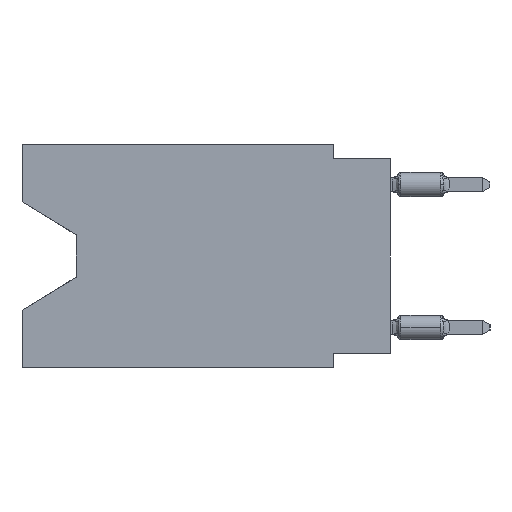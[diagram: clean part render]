
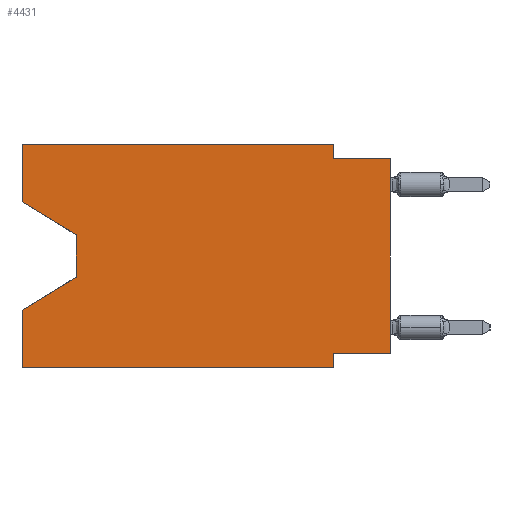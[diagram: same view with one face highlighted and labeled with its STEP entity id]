
A CAD part, left-side view. The second image highlights one B-rep face of the part: STEP entity #4431.
In plain terms, the highlighted planar face has unit normal (-1, 0, 0).
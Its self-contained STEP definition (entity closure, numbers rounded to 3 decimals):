
#127 = ORIENTED_EDGE ( 'NONE', *, *, #1039, .T. ) ;
#1039 = EDGE_CURVE ( 'NONE', #34887, #13111, #49530, .T. ) ;
#1894 = VERTEX_POINT ( 'NONE', #21751 ) ;
#2171 = EDGE_LOOP ( 'NONE', ( #127, #11190, #15120, #26496, #33015, #48427, #23847, #25367, #46181, #34210, #42663, #42930 ) ) ;
#2416 = DIRECTION ( 'NONE',  ( 1., 0., 0. ) ) ;
#3726 = DIRECTION ( 'NONE',  ( 0., -1., 0. ) ) ;
#3860 = VERTEX_POINT ( 'NONE', #38216 ) ;
#4060 = CARTESIAN_POINT ( 'NONE',  ( 0., 13.97, -4.013 ) ) ;
#4105 = CARTESIAN_POINT ( 'NONE',  ( 0., 2.54, -9.906 ) ) ;
#4187 = VECTOR ( 'NONE', #3726, 1000. ) ;
#4391 = VECTOR ( 'NONE', #30835, 1000. ) ;
#4431 = ADVANCED_FACE ( 'NONE', ( #23370 ), #11126, .F. ) ;
#4784 = CARTESIAN_POINT ( 'NONE',  ( 0., 13.97, -4.013 ) ) ;
#5749 = VECTOR ( 'NONE', #38056, 1000. ) ;
#6644 = DIRECTION ( 'NONE',  ( 0., -1., 0. ) ) ;
#7010 = LINE ( 'NONE', #11376, #11803 ) ;
#7080 = EDGE_CURVE ( 'NONE', #3860, #18560, #20617, .T. ) ;
#8147 = DIRECTION ( 'NONE',  ( 0., -0.855, -0.519 ) ) ;
#8660 = DIRECTION ( 'NONE',  ( 0., 0., -1. ) ) ;
#9831 = CARTESIAN_POINT ( 'NONE',  ( 0., 0., -0.635 ) ) ;
#10659 = EDGE_CURVE ( 'NONE', #34887, #3860, #22140, .T. ) ;
#11126 = PLANE ( 'NONE',  #47541 ) ;
#11190 = ORIENTED_EDGE ( 'NONE', *, *, #38778, .T. ) ;
#11282 = CARTESIAN_POINT ( 'NONE',  ( 0., 16.383, -9.906 ) ) ;
#11376 = CARTESIAN_POINT ( 'NONE',  ( 0., 16.383, 0. ) ) ;
#11718 = LINE ( 'NONE', #4060, #34332 ) ;
#11803 = VECTOR ( 'NONE', #48397, 1000. ) ;
#11830 = VECTOR ( 'NONE', #6644, 1000. ) ;
#12264 = VERTEX_POINT ( 'NONE', #4105 ) ;
#12489 = LINE ( 'NONE', #20931, #5749 ) ;
#13111 = VERTEX_POINT ( 'NONE', #4784 ) ;
#13801 = VERTEX_POINT ( 'NONE', #52596 ) ;
#14171 = EDGE_CURVE ( 'NONE', #26111, #46041, #38941, .T. ) ;
#15120 = ORIENTED_EDGE ( 'NONE', *, *, #14171, .T. ) ;
#15475 = CARTESIAN_POINT ( 'NONE',  ( 0., 16.383, 0. ) ) ;
#15873 = LINE ( 'NONE', #32461, #23120 ) ;
#16841 = CARTESIAN_POINT ( 'NONE',  ( 0., 2.54, -9.906 ) ) ;
#17109 = LINE ( 'NONE', #16841, #31672 ) ;
#17131 = EDGE_CURVE ( 'NONE', #46244, #46041, #7010, .T. ) ;
#17999 = DIRECTION ( 'NONE',  ( 0., 0.855, -0.519 ) ) ;
#18350 = EDGE_CURVE ( 'NONE', #13801, #36862, #33402, .T. ) ;
#18560 = VERTEX_POINT ( 'NONE', #50554 ) ;
#19128 = EDGE_CURVE ( 'NONE', #46244, #12264, #44469, .T. ) ;
#20617 = LINE ( 'NONE', #49985, #4187 ) ;
#20931 = CARTESIAN_POINT ( 'NONE',  ( 0., 2.54, 0. ) ) ;
#20972 = VERTEX_POINT ( 'NONE', #25330 ) ;
#21751 = CARTESIAN_POINT ( 'NONE',  ( 0., 2.54, -0.635 ) ) ;
#22140 = LINE ( 'NONE', #43083, #4391 ) ;
#23120 = VECTOR ( 'NONE', #29983, 1000. ) ;
#23370 = FACE_OUTER_BOUND ( 'NONE', #2171, .T. ) ;
#23739 = VECTOR ( 'NONE', #8147, 1000. ) ;
#23847 = ORIENTED_EDGE ( 'NONE', *, *, #39685, .F. ) ;
#23990 = CARTESIAN_POINT ( 'NONE',  ( 0., 16.383, -9.906 ) ) ;
#25330 = CARTESIAN_POINT ( 'NONE',  ( 0., 2.54, -9.271 ) ) ;
#25367 = ORIENTED_EDGE ( 'NONE', *, *, #18350, .T. ) ;
#25546 = CARTESIAN_POINT ( 'NONE',  ( 0., 0., -0.635 ) ) ;
#26111 = VERTEX_POINT ( 'NONE', #52553 ) ;
#26496 = ORIENTED_EDGE ( 'NONE', *, *, #17131, .F. ) ;
#26695 = LINE ( 'NONE', #9831, #41961 ) ;
#26961 = DIRECTION ( 'NONE',  ( 0., -1., 0. ) ) ;
#29853 = EDGE_CURVE ( 'NONE', #1894, #36862, #26695, .T. ) ;
#29983 = DIRECTION ( 'NONE',  ( 0., 1., 0. ) ) ;
#30223 = CARTESIAN_POINT ( 'NONE',  ( 0., 13.97, -5.893 ) ) ;
#30835 = DIRECTION ( 'NONE',  ( 0., 0., 1. ) ) ;
#31672 = VECTOR ( 'NONE', #8660, 1000. ) ;
#32461 = CARTESIAN_POINT ( 'NONE',  ( 0., 0., -9.271 ) ) ;
#32605 = CARTESIAN_POINT ( 'NONE',  ( 0., 0., 0. ) ) ;
#33015 = ORIENTED_EDGE ( 'NONE', *, *, #19128, .T. ) ;
#33178 = CARTESIAN_POINT ( 'NONE',  ( 0., 16.383, -2.546 ) ) ;
#33275 = CARTESIAN_POINT ( 'NONE',  ( 0., 16.383, -7.36 ) ) ;
#33402 = LINE ( 'NONE', #32605, #50920 ) ;
#33812 = EDGE_CURVE ( 'NONE', #20972, #12264, #17109, .T. ) ;
#34210 = ORIENTED_EDGE ( 'NONE', *, *, #35596, .F. ) ;
#34332 = VECTOR ( 'NONE', #49003, 1000. ) ;
#34887 = VERTEX_POINT ( 'NONE', #47721 ) ;
#35596 = EDGE_CURVE ( 'NONE', #18560, #1894, #12489, .T. ) ;
#36862 = VERTEX_POINT ( 'NONE', #25546 ) ;
#38056 = DIRECTION ( 'NONE',  ( 0., 0., -1. ) ) ;
#38216 = CARTESIAN_POINT ( 'NONE',  ( 0., 16.383, 0. ) ) ;
#38778 = EDGE_CURVE ( 'NONE', #13111, #26111, #11718, .T. ) ;
#38941 = LINE ( 'NONE', #30223, #42895 ) ;
#39685 = EDGE_CURVE ( 'NONE', #13801, #20972, #15873, .T. ) ;
#40485 = DIRECTION ( 'NONE',  ( 0., 0., -1. ) ) ;
#41576 = DIRECTION ( 'NONE',  ( 0., 0., 1. ) ) ;
#41961 = VECTOR ( 'NONE', #26961, 1000. ) ;
#42663 = ORIENTED_EDGE ( 'NONE', *, *, #7080, .F. ) ;
#42895 = VECTOR ( 'NONE', #17999, 1000. ) ;
#42930 = ORIENTED_EDGE ( 'NONE', *, *, #10659, .F. ) ;
#43083 = CARTESIAN_POINT ( 'NONE',  ( 0., 16.383, 0. ) ) ;
#44469 = LINE ( 'NONE', #11282, #11830 ) ;
#46041 = VERTEX_POINT ( 'NONE', #33275 ) ;
#46181 = ORIENTED_EDGE ( 'NONE', *, *, #29853, .F. ) ;
#46244 = VERTEX_POINT ( 'NONE', #23990 ) ;
#47541 = AXIS2_PLACEMENT_3D ( 'NONE', #15475, #2416, #40485 ) ;
#47721 = CARTESIAN_POINT ( 'NONE',  ( 0., 16.383, -2.546 ) ) ;
#48397 = DIRECTION ( 'NONE',  ( 0., 0., 1. ) ) ;
#48427 = ORIENTED_EDGE ( 'NONE', *, *, #33812, .F. ) ;
#49003 = DIRECTION ( 'NONE',  ( 0., 0., -1. ) ) ;
#49530 = LINE ( 'NONE', #33178, #23739 ) ;
#49985 = CARTESIAN_POINT ( 'NONE',  ( 0., 16.383, 0. ) ) ;
#50554 = CARTESIAN_POINT ( 'NONE',  ( 0., 2.54, 0. ) ) ;
#50920 = VECTOR ( 'NONE', #41576, 1000. ) ;
#52553 = CARTESIAN_POINT ( 'NONE',  ( 0., 13.97, -5.893 ) ) ;
#52596 = CARTESIAN_POINT ( 'NONE',  ( 0., 0., -9.271 ) ) ;
